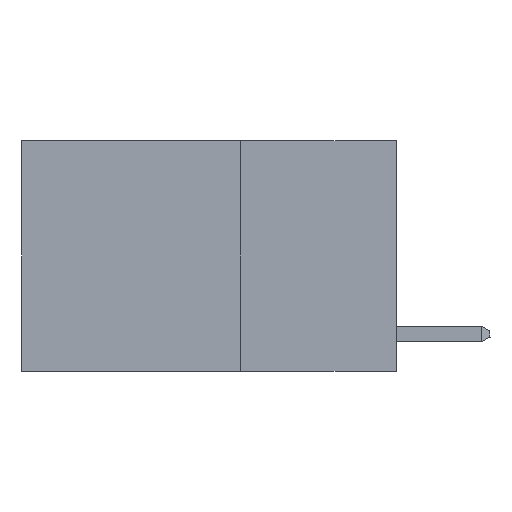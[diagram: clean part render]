
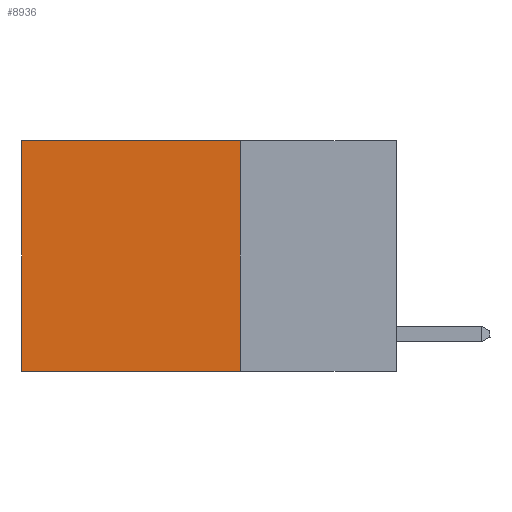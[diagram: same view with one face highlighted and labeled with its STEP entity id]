
A CAD part, left-side view. The second image highlights one B-rep face of the part: STEP entity #8936.
In plain terms, the highlighted planar face has unit normal (-1, 0, 0).
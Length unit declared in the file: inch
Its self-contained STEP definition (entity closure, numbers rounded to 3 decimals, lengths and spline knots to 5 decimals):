
#488 = ORIENTED_EDGE ( 'NONE', *, *, #7562, .T. ) ;
#872 = VECTOR ( 'NONE', #10673, 39.37008 ) ;
#1949 = ORIENTED_EDGE ( 'NONE', *, *, #7843, .T. ) ;
#1987 = EDGE_CURVE ( 'NONE', #15151, #4182, #18400, .T. ) ;
#2042 = CARTESIAN_POINT ( 'NONE',  ( 0.2625, 0.25, 0. ) ) ;
#4182 = VERTEX_POINT ( 'NONE', #17341 ) ;
#4184 = CARTESIAN_POINT ( 'NONE',  ( 0.2625, 0.6, -0.37 ) ) ;
#4710 = DIRECTION ( 'NONE',  ( 1., 0., 0. ) ) ;
#4885 = LINE ( 'NONE', #14370, #17618 ) ;
#4965 = CARTESIAN_POINT ( 'NONE',  ( 0.2625, 0.25, 0. ) ) ;
#5188 = DIRECTION ( 'NONE',  ( 0., 1., 0. ) ) ;
#5570 = EDGE_CURVE ( 'NONE', #4182, #17531, #4885, .T. ) ;
#5964 = ORIENTED_EDGE ( 'NONE', *, *, #1987, .F. ) ;
#6594 = ORIENTED_EDGE ( 'NONE', *, *, #5570, .F. ) ;
#7562 = EDGE_CURVE ( 'NONE', #12985, #17531, #13163, .T. ) ;
#7843 = EDGE_CURVE ( 'NONE', #15151, #12985, #7900, .T. ) ;
#7881 = AXIS2_PLACEMENT_3D ( 'NONE', #12326, #4710, #15463 ) ;
#7900 = LINE ( 'NONE', #2042, #19674 ) ;
#8936 = ADVANCED_FACE ( 'NONE', ( #11932 ), #18463, .F. ) ;
#9125 = CARTESIAN_POINT ( 'NONE',  ( 0.2625, 0.6, 0. ) ) ;
#10569 = CARTESIAN_POINT ( 'NONE',  ( 0.2625, 0.25, 0. ) ) ;
#10673 = DIRECTION ( 'NONE',  ( 0., 0., -1. ) ) ;
#10726 = VECTOR ( 'NONE', #14145, 39.37008 ) ;
#11776 = CARTESIAN_POINT ( 'NONE',  ( 0.2625, 0.6, 0. ) ) ;
#11932 = FACE_OUTER_BOUND ( 'NONE', #13921, .T. ) ;
#12326 = CARTESIAN_POINT ( 'NONE',  ( 0.2625, 0.25, 0. ) ) ;
#12771 = DIRECTION ( 'NONE',  ( 0., 1., 0. ) ) ;
#12985 = VERTEX_POINT ( 'NONE', #11776 ) ;
#13163 = LINE ( 'NONE', #9125, #872 ) ;
#13921 = EDGE_LOOP ( 'NONE', ( #488, #6594, #5964, #1949 ) ) ;
#14145 = DIRECTION ( 'NONE',  ( 0., 0., -1. ) ) ;
#14370 = CARTESIAN_POINT ( 'NONE',  ( 0.2625, 0.25, -0.37 ) ) ;
#15151 = VERTEX_POINT ( 'NONE', #10569 ) ;
#15463 = DIRECTION ( 'NONE',  ( 0., 0., -1. ) ) ;
#17341 = CARTESIAN_POINT ( 'NONE',  ( 0.2625, 0.25, -0.37 ) ) ;
#17531 = VERTEX_POINT ( 'NONE', #4184 ) ;
#17618 = VECTOR ( 'NONE', #5188, 39.37008 ) ;
#18400 = LINE ( 'NONE', #4965, #10726 ) ;
#18463 = PLANE ( 'NONE',  #7881 ) ;
#19674 = VECTOR ( 'NONE', #12771, 39.37008 ) ;
